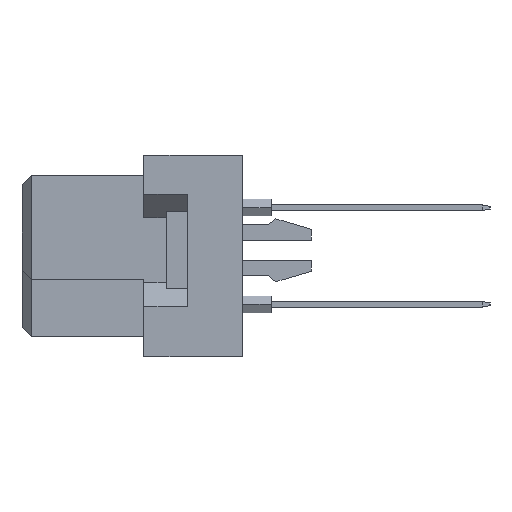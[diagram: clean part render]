
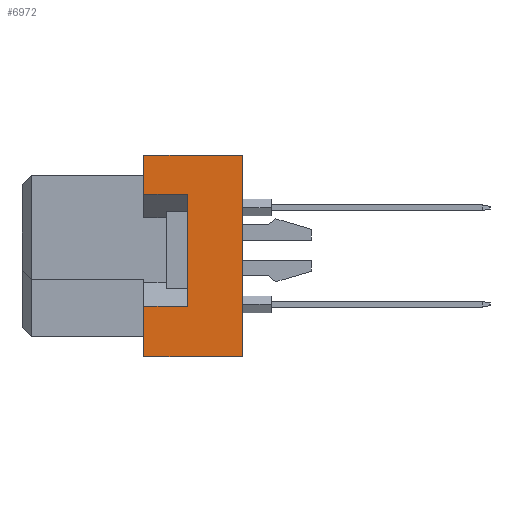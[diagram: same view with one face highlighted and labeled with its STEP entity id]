
A CAD part, left-side view. The second image highlights one B-rep face of the part: STEP entity #6972.
In plain terms, the highlighted planar face has unit normal (-1, 0, 0).
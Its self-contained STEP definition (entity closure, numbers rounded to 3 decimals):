
#116 = ORIENTED_EDGE ( 'NONE', *, *, #7850, .T. ) ;
#522 = DIRECTION ( 'NONE',  ( 0., 0., 1. ) ) ;
#1288 = DIRECTION ( 'NONE',  ( 0., 0., 1. ) ) ;
#2174 = FACE_OUTER_BOUND ( 'NONE', #38215, .T. ) ;
#2240 = VECTOR ( 'NONE', #28161, 1000. ) ;
#3032 = CARTESIAN_POINT ( 'NONE',  ( -47.5, -11.6, 5.3 ) ) ;
#3161 = VECTOR ( 'NONE', #1288, 1000. ) ;
#3785 = LINE ( 'NONE', #22738, #8324 ) ;
#3806 = EDGE_CURVE ( 'NONE', #24566, #30592, #38281, .T. ) ;
#5190 = VERTEX_POINT ( 'NONE', #36197 ) ;
#6744 = CARTESIAN_POINT ( 'NONE',  ( -47.5, -6.4, 3.25 ) ) ;
#6972 = ADVANCED_FACE ( 'NONE', ( #2174 ), #33684, .T. ) ;
#7595 = CARTESIAN_POINT ( 'NONE',  ( -47.5, -8.7, -2.65 ) ) ;
#7739 = VECTOR ( 'NONE', #37810, 1000. ) ;
#7751 = DIRECTION ( 'NONE',  ( -1., 0., 0. ) ) ;
#7850 = EDGE_CURVE ( 'NONE', #19394, #5190, #37697, .T. ) ;
#8037 = EDGE_CURVE ( 'NONE', #13990, #30592, #18239, .T. ) ;
#8324 = VECTOR ( 'NONE', #35303, 1000. ) ;
#9275 = DIRECTION ( 'NONE',  ( 0., 1., 0. ) ) ;
#9431 = LINE ( 'NONE', #3032, #2240 ) ;
#9499 = DIRECTION ( 'NONE',  ( 0., 0., 1. ) ) ;
#9604 = CARTESIAN_POINT ( 'NONE',  ( -47.5, -6.4, -5.3 ) ) ;
#11228 = EDGE_CURVE ( 'NONE', #19394, #13990, #21615, .T. ) ;
#12045 = VECTOR ( 'NONE', #9499, 1000. ) ;
#13923 = ORIENTED_EDGE ( 'NONE', *, *, #14971, .F. ) ;
#13990 = VERTEX_POINT ( 'NONE', #21077 ) ;
#14751 = CARTESIAN_POINT ( 'NONE',  ( -47.5, -11.6, 5.3 ) ) ;
#14755 = LINE ( 'NONE', #26199, #3161 ) ;
#14971 = EDGE_CURVE ( 'NONE', #28000, #22443, #28345, .T. ) ;
#16588 = ORIENTED_EDGE ( 'NONE', *, *, #37744, .T. ) ;
#16660 = DIRECTION ( 'NONE',  ( 0., 1., 0. ) ) ;
#16691 = ORIENTED_EDGE ( 'NONE', *, *, #11228, .F. ) ;
#18239 = LINE ( 'NONE', #28543, #7739 ) ;
#18855 = CARTESIAN_POINT ( 'NONE',  ( -47.5, -6.4, -2.65 ) ) ;
#19394 = VERTEX_POINT ( 'NONE', #37718 ) ;
#20122 = CARTESIAN_POINT ( 'NONE',  ( -47.5, -11.6, 5.3 ) ) ;
#21077 = CARTESIAN_POINT ( 'NONE',  ( -47.5, -6.4, -5.3 ) ) ;
#21615 = LINE ( 'NONE', #37469, #27574 ) ;
#22443 = VERTEX_POINT ( 'NONE', #26680 ) ;
#22738 = CARTESIAN_POINT ( 'NONE',  ( -47.5, -8.7, 3.25 ) ) ;
#23196 = ORIENTED_EDGE ( 'NONE', *, *, #26719, .F. ) ;
#24566 = VERTEX_POINT ( 'NONE', #34781 ) ;
#26199 = CARTESIAN_POINT ( 'NONE',  ( -47.5, -8.7, -2.65 ) ) ;
#26680 = CARTESIAN_POINT ( 'NONE',  ( -47.5, -6.4, 5.3 ) ) ;
#26719 = EDGE_CURVE ( 'NONE', #36792, #28000, #3785, .T. ) ;
#26811 = ORIENTED_EDGE ( 'NONE', *, *, #3806, .T. ) ;
#26889 = DIRECTION ( 'NONE',  ( 0., 0., 1. ) ) ;
#27484 = CARTESIAN_POINT ( 'NONE',  ( -47.5, -8.7, 3.25 ) ) ;
#27574 = VECTOR ( 'NONE', #9275, 1000. ) ;
#28000 = VERTEX_POINT ( 'NONE', #6744 ) ;
#28161 = DIRECTION ( 'NONE',  ( 0., 1., 0. ) ) ;
#28277 = EDGE_CURVE ( 'NONE', #24566, #36792, #14755, .T. ) ;
#28345 = LINE ( 'NONE', #9604, #36880 ) ;
#28543 = CARTESIAN_POINT ( 'NONE',  ( -47.5, -6.4, -5.3 ) ) ;
#29690 = AXIS2_PLACEMENT_3D ( 'NONE', #14751, #7751, #26889 ) ;
#30592 = VERTEX_POINT ( 'NONE', #18855 ) ;
#31060 = ORIENTED_EDGE ( 'NONE', *, *, #8037, .F. ) ;
#33684 = PLANE ( 'NONE',  #29690 ) ;
#34781 = CARTESIAN_POINT ( 'NONE',  ( -47.5, -8.7, -2.65 ) ) ;
#35303 = DIRECTION ( 'NONE',  ( 0., 1., 0. ) ) ;
#36197 = CARTESIAN_POINT ( 'NONE',  ( -47.5, -11.6, 5.3 ) ) ;
#36792 = VERTEX_POINT ( 'NONE', #27484 ) ;
#36880 = VECTOR ( 'NONE', #522, 1000. ) ;
#37422 = VECTOR ( 'NONE', #16660, 1000. ) ;
#37469 = CARTESIAN_POINT ( 'NONE',  ( -47.5, -11.6, -5.3 ) ) ;
#37697 = LINE ( 'NONE', #20122, #12045 ) ;
#37718 = CARTESIAN_POINT ( 'NONE',  ( -47.5, -11.6, -5.3 ) ) ;
#37744 = EDGE_CURVE ( 'NONE', #5190, #22443, #9431, .T. ) ;
#37810 = DIRECTION ( 'NONE',  ( 0., 0., 1. ) ) ;
#38215 = EDGE_LOOP ( 'NONE', ( #26811, #31060, #16691, #116, #16588, #13923, #23196, #38726 ) ) ;
#38281 = LINE ( 'NONE', #7595, #37422 ) ;
#38726 = ORIENTED_EDGE ( 'NONE', *, *, #28277, .F. ) ;
